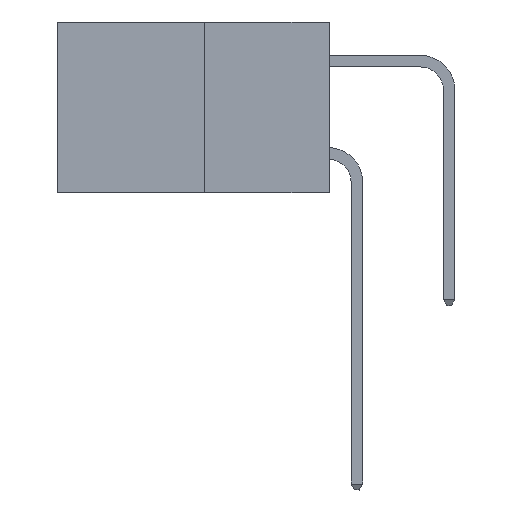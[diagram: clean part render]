
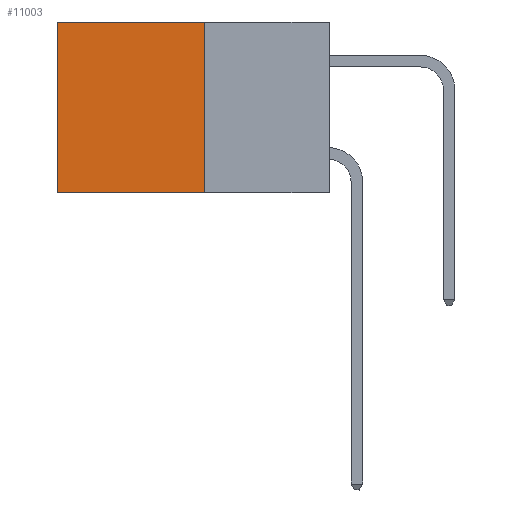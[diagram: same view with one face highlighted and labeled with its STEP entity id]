
A CAD part, left-side view. The second image highlights one B-rep face of the part: STEP entity #11003.
In plain terms, the highlighted planar face has unit normal (-1, 0, 0).
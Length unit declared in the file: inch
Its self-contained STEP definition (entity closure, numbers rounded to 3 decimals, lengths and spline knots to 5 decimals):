
#561 = VERTEX_POINT ( 'NONE', #4860 ) ;
#3037 = ORIENTED_EDGE ( 'NONE', *, *, #23406, .T. ) ;
#3537 = ORIENTED_EDGE ( 'NONE', *, *, #30975, .F. ) ;
#4238 = CARTESIAN_POINT ( 'NONE',  ( 0.277, 0.27, -0.37 ) ) ;
#4412 = DIRECTION ( 'NONE',  ( 0., 0., -1. ) ) ;
#4860 = CARTESIAN_POINT ( 'NONE',  ( 0.277, 0.59, 0. ) ) ;
#6080 = VECTOR ( 'NONE', #24203, 39.37008 ) ;
#7009 = CARTESIAN_POINT ( 'NONE',  ( 0.277, 0.27, -0.37 ) ) ;
#7338 = ORIENTED_EDGE ( 'NONE', *, *, #30188, .F. ) ;
#7860 = VERTEX_POINT ( 'NONE', #4238 ) ;
#8390 = VECTOR ( 'NONE', #14424, 39.37008 ) ;
#9384 = EDGE_LOOP ( 'NONE', ( #10962, #3537, #7338, #3037 ) ) ;
#10962 = ORIENTED_EDGE ( 'NONE', *, *, #30802, .T. ) ;
#11003 = ADVANCED_FACE ( 'NONE', ( #30005 ), #23696, .F. ) ;
#11413 = LINE ( 'NONE', #30843, #24193 ) ;
#11465 = LINE ( 'NONE', #14176, #29119 ) ;
#13829 = AXIS2_PLACEMENT_3D ( 'NONE', #14177, #30891, #16639 ) ;
#14125 = DIRECTION ( 'NONE',  ( 0., 1., 0. ) ) ;
#14176 = CARTESIAN_POINT ( 'NONE',  ( 0.277, 0.59, -0.37 ) ) ;
#14177 = CARTESIAN_POINT ( 'NONE',  ( 0.277, 0.27, -0.37 ) ) ;
#14424 = DIRECTION ( 'NONE',  ( 0., 0., -1. ) ) ;
#16639 = DIRECTION ( 'NONE',  ( 0., 0., -1. ) ) ;
#17177 = CARTESIAN_POINT ( 'NONE',  ( 0.277, 0.27, -0.37 ) ) ;
#18159 = CARTESIAN_POINT ( 'NONE',  ( 0.277, 0.59, -0.37 ) ) ;
#20623 = VERTEX_POINT ( 'NONE', #29592 ) ;
#23406 = EDGE_CURVE ( 'NONE', #20623, #561, #11413, .T. ) ;
#23696 = PLANE ( 'NONE',  #13829 ) ;
#24193 = VECTOR ( 'NONE', #14125, 39.37008 ) ;
#24203 = DIRECTION ( 'NONE',  ( 0., 1., 0. ) ) ;
#25066 = VERTEX_POINT ( 'NONE', #18159 ) ;
#26088 = LINE ( 'NONE', #17177, #6080 ) ;
#26843 = LINE ( 'NONE', #7009, #8390 ) ;
#29119 = VECTOR ( 'NONE', #4412, 39.37008 ) ;
#29592 = CARTESIAN_POINT ( 'NONE',  ( 0.277, 0.27, 0. ) ) ;
#30005 = FACE_OUTER_BOUND ( 'NONE', #9384, .T. ) ;
#30188 = EDGE_CURVE ( 'NONE', #20623, #7860, #26843, .T. ) ;
#30802 = EDGE_CURVE ( 'NONE', #561, #25066, #11465, .T. ) ;
#30843 = CARTESIAN_POINT ( 'NONE',  ( 0.277, 0.27, 0. ) ) ;
#30891 = DIRECTION ( 'NONE',  ( 1., 0., 0. ) ) ;
#30975 = EDGE_CURVE ( 'NONE', #7860, #25066, #26088, .T. ) ;
